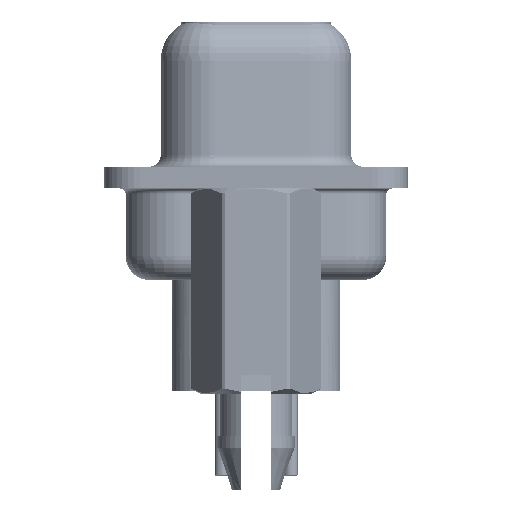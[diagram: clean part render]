
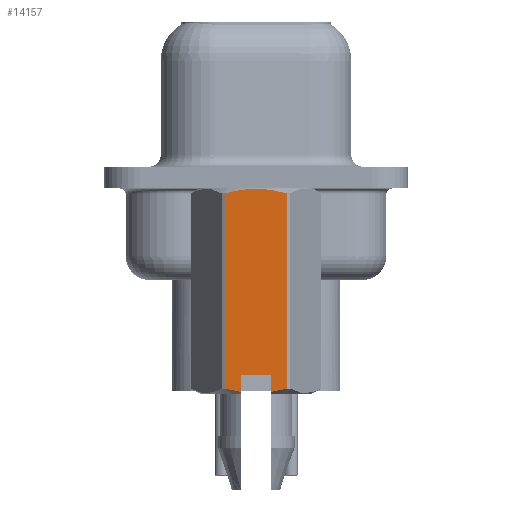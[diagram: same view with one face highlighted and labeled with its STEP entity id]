
A CAD part, left-side view. The second image highlights one B-rep face of the part: STEP entity #14157.
In plain terms, the highlighted planar face has unit normal (-1, 0, 0).
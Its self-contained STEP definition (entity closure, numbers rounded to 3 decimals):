
#891 = VERTEX_POINT ( 'NONE', #19298 ) ;
#3489 = VECTOR ( 'NONE', #31351, 1000. ) ;
#3873 = DIRECTION ( 'NONE',  ( 0., 1., 0. ) ) ;
#4119 = EDGE_CURVE ( 'NONE', #32352, #16789, #21928, .T. ) ;
#4586 = ORIENTED_EDGE ( 'NONE', *, *, #4119, .T. ) ;
#5784 = AXIS2_PLACEMENT_3D ( 'NONE', #38162, #19140, #18406 ) ;
#6293 = CARTESIAN_POINT ( 'NONE',  ( -2.381, -0.215, -0.468 ) ) ;
#6505 = CARTESIAN_POINT ( 'NONE',  ( -2.381, -0.625, -8.2 ) ) ;
#6762 = DIRECTION ( 'NONE',  ( 0., 0., -1. ) ) ;
#6919 = CARTESIAN_POINT ( 'NONE',  ( -2.381, -0.842, -8.854 ) ) ;
#7343 = CARTESIAN_POINT ( 'NONE',  ( -2.381, 1.06, -8.806 ) ) ;
#7524 = VECTOR ( 'NONE', #34396, 1000. ) ;
#8845 = LINE ( 'NONE', #38179, #24268 ) ;
#9626 = ORIENTED_EDGE ( 'NONE', *, *, #43937, .T. ) ;
#9911 = CARTESIAN_POINT ( 'NONE',  ( -2.381, -1.273, -8.748 ) ) ;
#9964 = EDGE_CURVE ( 'NONE', #40113, #21401, #8845, .T. ) ;
#10045 = CARTESIAN_POINT ( 'NONE',  ( -2.381, -1.065, -0.596 ) ) ;
#10109 = CARTESIAN_POINT ( 'NONE',  ( -2.381, 1.273, -8.748 ) ) ;
#10859 = VECTOR ( 'NONE', #6762, 1000. ) ;
#12737 = ORIENTED_EDGE ( 'NONE', *, *, #40834, .T. ) ;
#13760 = CARTESIAN_POINT ( 'NONE',  ( -2.381, 0.215, -0.468 ) ) ;
#14010 = LINE ( 'NONE', #6505, #10859 ) ;
#14157 = ADVANCED_FACE ( 'NONE', ( #18906 ), #15126, .T. ) ;
#14168 = CARTESIAN_POINT ( 'NONE',  ( -2.381, -0.625, -8.2 ) ) ;
#14508 = CARTESIAN_POINT ( 'NONE',  ( -2.381, -1.273, 0.581 ) ) ;
#15126 = PLANE ( 'NONE',  #5784 ) ;
#16077 = CARTESIAN_POINT ( 'NONE',  ( -2.381, 1.273, 0.581 ) ) ;
#16789 = VERTEX_POINT ( 'NONE', #47038 ) ;
#18395 = CARTESIAN_POINT ( 'NONE',  ( -2.381, 0.625, -8.2 ) ) ;
#18406 = DIRECTION ( 'NONE',  ( 0., 0., 1. ) ) ;
#18906 = FACE_OUTER_BOUND ( 'NONE', #44105, .T. ) ;
#19140 = DIRECTION ( 'NONE',  ( -1., 0., 0. ) ) ;
#19298 = CARTESIAN_POINT ( 'NONE',  ( -2.381, -1.273, -8.748 ) ) ;
#21183 = CARTESIAN_POINT ( 'NONE',  ( -2.381, -0.625, -8.885 ) ) ;
#21401 = VERTEX_POINT ( 'NONE', #38992 ) ;
#21557 = CARTESIAN_POINT ( 'NONE',  ( -2.381, 0., -0.468 ) ) ;
#21928 = B_SPLINE_CURVE_WITH_KNOTS ( 'NONE', 3,
 ( #33074, #10045, #33326, #40587, #6293, #21557 ),
 .UNSPECIFIED., .F., .F.,
 ( 4, 2, 4 ),
 ( 0.003, 0.003, 0.004 ),
 .UNSPECIFIED. ) ;
#22077 = EDGE_CURVE ( 'NONE', #40529, #25750, #26156, .T. ) ;
#22519 = B_SPLINE_CURVE_WITH_KNOTS ( 'NONE', 3,
 ( #21183, #6919, #36473, #9911 ),
 .UNSPECIFIED., .F., .F.,
 ( 4, 4 ),
 ( 0.003, 0.004 ),
 .UNSPECIFIED. ) ;
#22523 = LINE ( 'NONE', #14508, #29752 ) ;
#22870 = CARTESIAN_POINT ( 'NONE',  ( -2.381, 0.845, -8.853 ) ) ;
#24268 = VECTOR ( 'NONE', #3873, 1000. ) ;
#25290 = CARTESIAN_POINT ( 'NONE',  ( -2.381, 0., -0.468 ) ) ;
#25750 = VERTEX_POINT ( 'NONE', #46981 ) ;
#25881 = ORIENTED_EDGE ( 'NONE', *, *, #36695, .T. ) ;
#26156 = B_SPLINE_CURVE_WITH_KNOTS ( 'NONE', 3,
 ( #10109, #7343, #22870, #37648 ),
 .UNSPECIFIED., .F., .F.,
 ( 4, 4 ),
 ( 0.001, 0.002 ),
 .UNSPECIFIED. ) ;
#26596 = CARTESIAN_POINT ( 'NONE',  ( -2.381, -0.625, -8.885 ) ) ;
#28585 = CARTESIAN_POINT ( 'NONE',  ( -2.381, -1.273, -0.652 ) ) ;
#28894 = EDGE_CURVE ( 'NONE', #45118, #891, #22519, .T. ) ;
#29752 = VECTOR ( 'NONE', #30299, 1000. ) ;
#30299 = DIRECTION ( 'NONE',  ( 0., 0., 1. ) ) ;
#31351 = DIRECTION ( 'NONE',  ( 0., 0., -1. ) ) ;
#31809 = CARTESIAN_POINT ( 'NONE',  ( -2.381, 0.858, -0.55 ) ) ;
#32300 = CARTESIAN_POINT ( 'NONE',  ( -2.381, 0.432, -0.485 ) ) ;
#32352 = VERTEX_POINT ( 'NONE', #28585 ) ;
#33074 = CARTESIAN_POINT ( 'NONE',  ( -2.381, -1.273, -0.652 ) ) ;
#33326 = CARTESIAN_POINT ( 'NONE',  ( -2.381, -0.853, -0.549 ) ) ;
#34396 = DIRECTION ( 'NONE',  ( 0., 0., -1. ) ) ;
#35110 = LINE ( 'NONE', #16077, #3489 ) ;
#35495 = ORIENTED_EDGE ( 'NONE', *, *, #9964, .F. ) ;
#36473 = CARTESIAN_POINT ( 'NONE',  ( -2.381, -1.06, -8.806 ) ) ;
#36695 = EDGE_CURVE ( 'NONE', #16789, #41595, #43016, .T. ) ;
#36883 = EDGE_CURVE ( 'NONE', #891, #32352, #22523, .T. ) ;
#37153 = ORIENTED_EDGE ( 'NONE', *, *, #28894, .T. ) ;
#37648 = CARTESIAN_POINT ( 'NONE',  ( -2.381, 0.625, -8.885 ) ) ;
#38134 = ORIENTED_EDGE ( 'NONE', *, *, #22077, .T. ) ;
#38162 = CARTESIAN_POINT ( 'NONE',  ( -2.381, -1.375, 7.399 ) ) ;
#38179 = CARTESIAN_POINT ( 'NONE',  ( -2.381, -0.625, -8.2 ) ) ;
#38992 = CARTESIAN_POINT ( 'NONE',  ( -2.381, 0.625, -8.2 ) ) ;
#40113 = VERTEX_POINT ( 'NONE', #14168 ) ;
#40529 = VERTEX_POINT ( 'NONE', #48653 ) ;
#40587 = CARTESIAN_POINT ( 'NONE',  ( -2.381, -0.428, -0.485 ) ) ;
#40834 = EDGE_CURVE ( 'NONE', #41595, #40529, #35110, .T. ) ;
#41595 = VERTEX_POINT ( 'NONE', #45945 ) ;
#42503 = EDGE_CURVE ( 'NONE', #21401, #25750, #48674, .T. ) ;
#43016 = B_SPLINE_CURVE_WITH_KNOTS ( 'NONE', 3,
 ( #25290, #13760, #32300, #31809, #47572, #47321 ),
 .UNSPECIFIED., .F., .F.,
 ( 4, 2, 4 ),
 ( 0.004, 0.004, 0.005 ),
 .UNSPECIFIED. ) ;
#43806 = ORIENTED_EDGE ( 'NONE', *, *, #42503, .F. ) ;
#43937 = EDGE_CURVE ( 'NONE', #40113, #45118, #14010, .T. ) ;
#44105 = EDGE_LOOP ( 'NONE', ( #43806, #35495, #9626, #37153, #45511, #4586, #25881, #12737, #38134 ) ) ;
#45118 = VERTEX_POINT ( 'NONE', #26596 ) ;
#45511 = ORIENTED_EDGE ( 'NONE', *, *, #36883, .T. ) ;
#45945 = CARTESIAN_POINT ( 'NONE',  ( -2.381, 1.273, -0.652 ) ) ;
#46981 = CARTESIAN_POINT ( 'NONE',  ( -2.381, 0.625, -8.885 ) ) ;
#47038 = CARTESIAN_POINT ( 'NONE',  ( -2.381, 0., -0.468 ) ) ;
#47321 = CARTESIAN_POINT ( 'NONE',  ( -2.381, 1.273, -0.652 ) ) ;
#47572 = CARTESIAN_POINT ( 'NONE',  ( -2.381, 1.066, -0.596 ) ) ;
#48653 = CARTESIAN_POINT ( 'NONE',  ( -2.381, 1.273, -8.748 ) ) ;
#48674 = LINE ( 'NONE', #18395, #7524 ) ;
